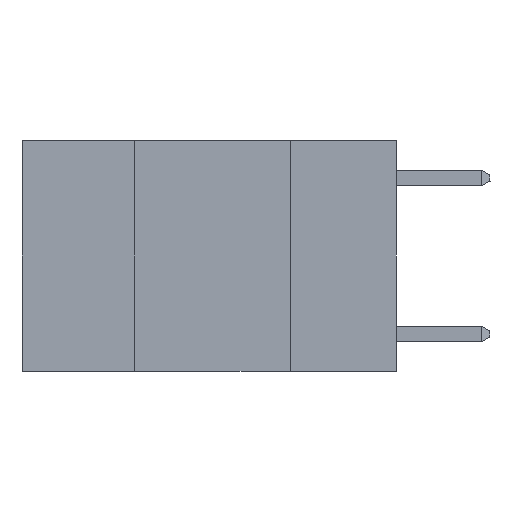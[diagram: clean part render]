
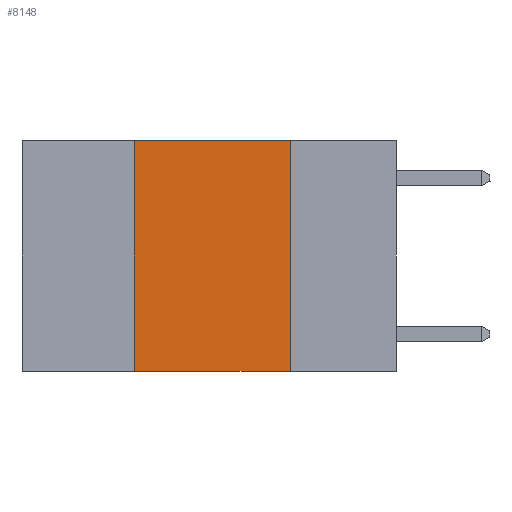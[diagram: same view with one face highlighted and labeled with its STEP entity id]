
A CAD part, left-side view. The second image highlights one B-rep face of the part: STEP entity #8148.
In plain terms, the highlighted planar face has unit normal (-1, 0, 0).
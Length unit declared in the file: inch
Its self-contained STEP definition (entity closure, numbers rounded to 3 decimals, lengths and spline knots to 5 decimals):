
#137 = ORIENTED_EDGE ( 'NONE', *, *, #5814, .F. ) ;
#301 = VERTEX_POINT ( 'NONE', #7171 ) ;
#495 = DIRECTION ( 'NONE',  ( 0., 0., -1. ) ) ;
#505 = DIRECTION ( 'NONE',  ( 1., 0., 0. ) ) ;
#527 = CARTESIAN_POINT ( 'NONE',  ( 0., 0.6, 0. ) ) ;
#725 = PLANE ( 'NONE',  #3627 ) ;
#738 = ORIENTED_EDGE ( 'NONE', *, *, #7687, .F. ) ;
#750 = VERTEX_POINT ( 'NONE', #4164 ) ;
#1695 = CARTESIAN_POINT ( 'NONE',  ( 0., 0.42, -0.37 ) ) ;
#1934 = ORIENTED_EDGE ( 'NONE', *, *, #7577, .F. ) ;
#3211 = EDGE_LOOP ( 'NONE', ( #137, #1934, #738, #9391 ) ) ;
#3445 = VERTEX_POINT ( 'NONE', #4742 ) ;
#3627 = AXIS2_PLACEMENT_3D ( 'NONE', #527, #505, #495 ) ;
#4001 = FACE_OUTER_BOUND ( 'NONE', #3211, .T. ) ;
#4164 = CARTESIAN_POINT ( 'NONE',  ( 0., 0.42, 0. ) ) ;
#4742 = CARTESIAN_POINT ( 'NONE',  ( 0., 0.17, -0.37 ) ) ;
#5226 = VECTOR ( 'NONE', #6271, 39.37008 ) ;
#5275 = LINE ( 'NONE', #6301, #5226 ) ;
#5507 = VECTOR ( 'NONE', #7369, 39.37008 ) ;
#5602 = LINE ( 'NONE', #7447, #5507 ) ;
#5814 = EDGE_CURVE ( 'NONE', #301, #3445, #9078, .T. ) ;
#6075 = EDGE_CURVE ( 'NONE', #8084, #3445, #8789, .T. ) ;
#6271 = DIRECTION ( 'NONE',  ( 0., 0., 1. ) ) ;
#6301 = CARTESIAN_POINT ( 'NONE',  ( 0., 0.42, 0. ) ) ;
#7171 = CARTESIAN_POINT ( 'NONE',  ( 0., 0.17, 0. ) ) ;
#7369 = DIRECTION ( 'NONE',  ( 0., -1., 0. ) ) ;
#7447 = CARTESIAN_POINT ( 'NONE',  ( 0., 0.6, 0. ) ) ;
#7577 = EDGE_CURVE ( 'NONE', #750, #301, #5602, .T. ) ;
#7687 = EDGE_CURVE ( 'NONE', #8084, #750, #5275, .T. ) ;
#8084 = VERTEX_POINT ( 'NONE', #1695 ) ;
#8148 = ADVANCED_FACE ( 'NONE', ( #4001 ), #725, .F. ) ;
#8269 = DIRECTION ( 'NONE',  ( 0., -1., 0. ) ) ;
#8373 = CARTESIAN_POINT ( 'NONE',  ( 0., 0.6, -0.37 ) ) ;
#8719 = VECTOR ( 'NONE', #8269, 39.37008 ) ;
#8789 = LINE ( 'NONE', #8373, #8719 ) ;
#9070 = VECTOR ( 'NONE', #9297, 39.37008 ) ;
#9078 = LINE ( 'NONE', #9451, #9070 ) ;
#9297 = DIRECTION ( 'NONE',  ( 0., 0., -1. ) ) ;
#9391 = ORIENTED_EDGE ( 'NONE', *, *, #6075, .T. ) ;
#9451 = CARTESIAN_POINT ( 'NONE',  ( 0., 0.17, 0. ) ) ;
